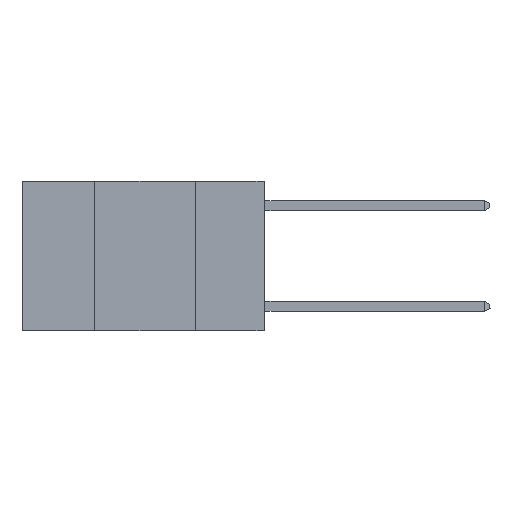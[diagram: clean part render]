
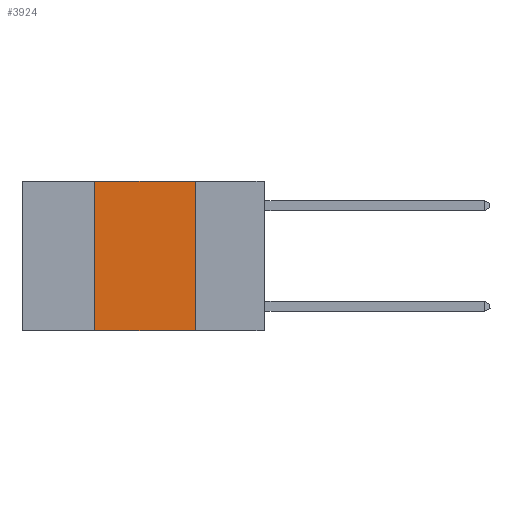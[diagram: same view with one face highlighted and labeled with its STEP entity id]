
A CAD part, left-side view. The second image highlights one B-rep face of the part: STEP entity #3924.
In plain terms, the highlighted planar face has unit normal (-1, 0, 0).
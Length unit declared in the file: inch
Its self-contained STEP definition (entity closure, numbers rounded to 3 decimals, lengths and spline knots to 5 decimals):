
#642 = VECTOR ( 'NONE', #6739, 39.37008 ) ;
#1187 = CARTESIAN_POINT ( 'NONE',  ( 0., 0.6, 0. ) ) ;
#1553 = LINE ( 'NONE', #1599, #6202 ) ;
#1599 = CARTESIAN_POINT ( 'NONE',  ( 0., 0.17, 0. ) ) ;
#1847 = CARTESIAN_POINT ( 'NONE',  ( 0., 0.42, -0.37 ) ) ;
#1896 = VERTEX_POINT ( 'NONE', #1847 ) ;
#2307 = ORIENTED_EDGE ( 'NONE', *, *, #6060, .F. ) ;
#2666 = DIRECTION ( 'NONE',  ( 0., -1., 0. ) ) ;
#2709 = CARTESIAN_POINT ( 'NONE',  ( 0., 0.6, -0.37 ) ) ;
#2910 = EDGE_CURVE ( 'NONE', #1896, #7333, #7991, .T. ) ;
#2984 = VECTOR ( 'NONE', #5397, 39.37008 ) ;
#3924 = ADVANCED_FACE ( 'NONE', ( #9860 ), #4674, .F. ) ;
#4425 = DIRECTION ( 'NONE',  ( 0., 0., -1. ) ) ;
#4438 = DIRECTION ( 'NONE',  ( 1., 0., 0. ) ) ;
#4650 = CARTESIAN_POINT ( 'NONE',  ( 0., 0.6, 0. ) ) ;
#4674 = PLANE ( 'NONE',  #6708 ) ;
#4818 = EDGE_CURVE ( 'NONE', #1896, #10515, #8174, .T. ) ;
#5217 = ORIENTED_EDGE ( 'NONE', *, *, #2910, .T. ) ;
#5280 = CARTESIAN_POINT ( 'NONE',  ( 0., 0.42, 0. ) ) ;
#5298 = EDGE_CURVE ( 'NONE', #11728, #7333, #1553, .T. ) ;
#5397 = DIRECTION ( 'NONE',  ( 0., 0., 1. ) ) ;
#6060 = EDGE_CURVE ( 'NONE', #10515, #11728, #8566, .T. ) ;
#6202 = VECTOR ( 'NONE', #6234, 39.37008 ) ;
#6234 = DIRECTION ( 'NONE',  ( 0., 0., -1. ) ) ;
#6708 = AXIS2_PLACEMENT_3D ( 'NONE', #4650, #4438, #4425 ) ;
#6739 = DIRECTION ( 'NONE',  ( 0., -1., 0. ) ) ;
#7108 = EDGE_LOOP ( 'NONE', ( #11106, #2307, #11528, #5217 ) ) ;
#7333 = VERTEX_POINT ( 'NONE', #9607 ) ;
#7991 = LINE ( 'NONE', #2709, #10362 ) ;
#8174 = LINE ( 'NONE', #9900, #2984 ) ;
#8566 = LINE ( 'NONE', #1187, #642 ) ;
#9607 = CARTESIAN_POINT ( 'NONE',  ( 0., 0.17, -0.37 ) ) ;
#9860 = FACE_OUTER_BOUND ( 'NONE', #7108, .T. ) ;
#9900 = CARTESIAN_POINT ( 'NONE',  ( 0., 0.42, 0. ) ) ;
#10362 = VECTOR ( 'NONE', #2666, 39.37008 ) ;
#10515 = VERTEX_POINT ( 'NONE', #5280 ) ;
#11106 = ORIENTED_EDGE ( 'NONE', *, *, #5298, .F. ) ;
#11487 = CARTESIAN_POINT ( 'NONE',  ( 0., 0.17, 0. ) ) ;
#11528 = ORIENTED_EDGE ( 'NONE', *, *, #4818, .F. ) ;
#11728 = VERTEX_POINT ( 'NONE', #11487 ) ;
